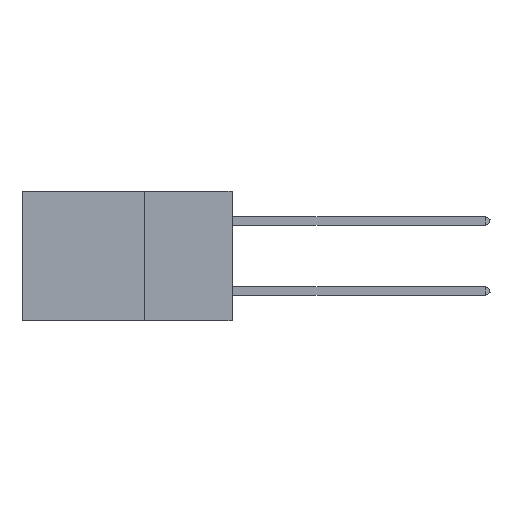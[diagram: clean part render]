
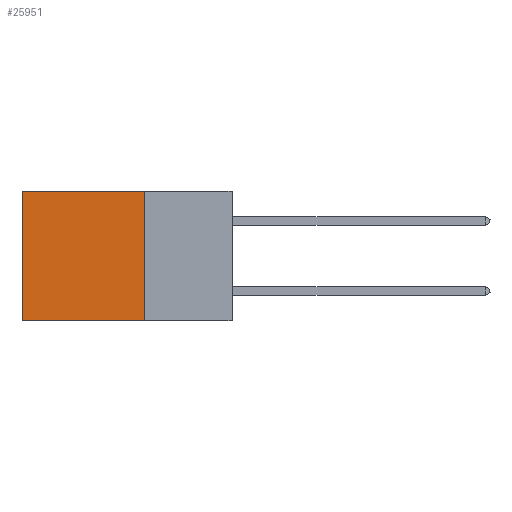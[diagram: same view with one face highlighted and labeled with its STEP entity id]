
A CAD part, left-side view. The second image highlights one B-rep face of the part: STEP entity #25951.
In plain terms, the highlighted planar face has unit normal (-1, 0, 0).
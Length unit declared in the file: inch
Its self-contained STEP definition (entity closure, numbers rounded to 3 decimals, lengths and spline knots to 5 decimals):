
#1373 = VECTOR ( 'NONE', #6215, 39.37008 ) ;
#1583 = EDGE_LOOP ( 'NONE', ( #2157, #2958, #23046, #15166 ) ) ;
#1660 = LINE ( 'NONE', #38741, #37101 ) ;
#2157 = ORIENTED_EDGE ( 'NONE', *, *, #16170, .T. ) ;
#2958 = ORIENTED_EDGE ( 'NONE', *, *, #44281, .F. ) ;
#4463 = VERTEX_POINT ( 'NONE', #35086 ) ;
#6215 = DIRECTION ( 'NONE',  ( 0., 1., 0. ) ) ;
#8748 = DIRECTION ( 'NONE',  ( 0., 0., -1. ) ) ;
#9686 = CARTESIAN_POINT ( 'NONE',  ( 0.2875, 0.25, 0. ) ) ;
#9754 = VERTEX_POINT ( 'NONE', #35437 ) ;
#10374 = VECTOR ( 'NONE', #38346, 39.37008 ) ;
#15166 = ORIENTED_EDGE ( 'NONE', *, *, #30765, .T. ) ;
#16008 = PLANE ( 'NONE',  #38828 ) ;
#16170 = EDGE_CURVE ( 'NONE', #22741, #35149, #24638, .T. ) ;
#17530 = EDGE_CURVE ( 'NONE', #9754, #4463, #46466, .T. ) ;
#22741 = VERTEX_POINT ( 'NONE', #38022 ) ;
#23046 = ORIENTED_EDGE ( 'NONE', *, *, #17530, .F. ) ;
#24638 = LINE ( 'NONE', #30742, #29705 ) ;
#25951 = ADVANCED_FACE ( 'NONE', ( #36941 ), #16008, .F. ) ;
#29705 = VECTOR ( 'NONE', #38464, 39.37008 ) ;
#30742 = CARTESIAN_POINT ( 'NONE',  ( 0.2875, 0.6, 0. ) ) ;
#30765 = EDGE_CURVE ( 'NONE', #9754, #22741, #31743, .T. ) ;
#30781 = DIRECTION ( 'NONE',  ( 1., 0., 0. ) ) ;
#31743 = LINE ( 'NONE', #35349, #1373 ) ;
#33051 = CARTESIAN_POINT ( 'NONE',  ( 0.2875, 0.6, -0.37 ) ) ;
#34562 = CARTESIAN_POINT ( 'NONE',  ( 0.2875, 0.25, 0. ) ) ;
#35086 = CARTESIAN_POINT ( 'NONE',  ( 0.2875, 0.25, -0.37 ) ) ;
#35149 = VERTEX_POINT ( 'NONE', #33051 ) ;
#35349 = CARTESIAN_POINT ( 'NONE',  ( 0.2875, 0.25, 0. ) ) ;
#35437 = CARTESIAN_POINT ( 'NONE',  ( 0.2875, 0.25, 0. ) ) ;
#36941 = FACE_OUTER_BOUND ( 'NONE', #1583, .T. ) ;
#37101 = VECTOR ( 'NONE', #45679, 39.37008 ) ;
#38022 = CARTESIAN_POINT ( 'NONE',  ( 0.2875, 0.6, 0. ) ) ;
#38346 = DIRECTION ( 'NONE',  ( 0., 0., -1. ) ) ;
#38464 = DIRECTION ( 'NONE',  ( 0., 0., -1. ) ) ;
#38741 = CARTESIAN_POINT ( 'NONE',  ( 0.2875, 0.25, -0.37 ) ) ;
#38828 = AXIS2_PLACEMENT_3D ( 'NONE', #34562, #30781, #8748 ) ;
#44281 = EDGE_CURVE ( 'NONE', #4463, #35149, #1660, .T. ) ;
#45679 = DIRECTION ( 'NONE',  ( 0., 1., 0. ) ) ;
#46466 = LINE ( 'NONE', #9686, #10374 ) ;
